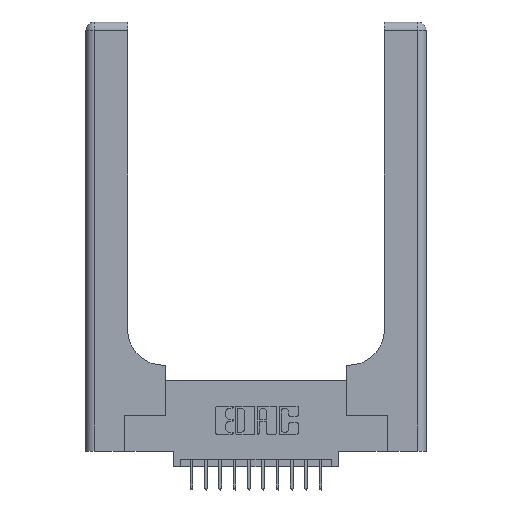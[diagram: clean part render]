
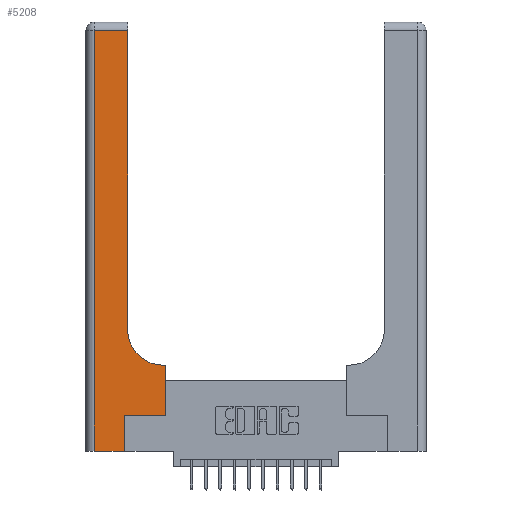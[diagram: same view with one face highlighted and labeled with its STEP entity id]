
A CAD part, top view. The second image highlights one B-rep face of the part: STEP entity #5208.
In plain terms, the highlighted planar face has unit normal (0, 0, 1).
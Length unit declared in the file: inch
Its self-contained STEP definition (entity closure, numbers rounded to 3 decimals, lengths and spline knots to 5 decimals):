
#75 = VERTEX_POINT ( 'NONE', #4749 ) ;
#174 = CARTESIAN_POINT ( 'NONE',  ( 0.5415, 0.6, 0.37 ) ) ;
#355 = PLANE ( 'NONE',  #7855 ) ;
#551 = CARTESIAN_POINT ( 'NONE',  ( 0.269, 0.25, 0.37 ) ) ;
#802 = EDGE_LOOP ( 'NONE', ( #6903, #7580, #8906, #9779, #12419, #13769, #14376, #15726, #12023 ) ) ;
#1086 = VERTEX_POINT ( 'NONE', #11250 ) ;
#1404 = EDGE_CURVE ( 'NONE', #2986, #9551, #2922, .T. ) ;
#1509 = CARTESIAN_POINT ( 'NONE',  ( 0.06, 2.94, 0.37 ) ) ;
#1578 = DIRECTION ( 'NONE',  ( -1., 0., 0. ) ) ;
#1774 = DIRECTION ( 'NONE',  ( 0., 0., -1. ) ) ;
#1851 = DIRECTION ( 'NONE',  ( 0., -1., 0. ) ) ;
#2357 = CARTESIAN_POINT ( 'NONE',  ( 0.2915, 2.94, 0.37 ) ) ;
#2883 = CARTESIAN_POINT ( 'NONE',  ( 0.269, 0.25, 0.37 ) ) ;
#2922 = LINE ( 'NONE', #15403, #3370 ) ;
#2986 = VERTEX_POINT ( 'NONE', #9006 ) ;
#3007 = LINE ( 'NONE', #17312, #10222 ) ;
#3303 = CARTESIAN_POINT ( 'NONE',  ( 0., 2.94, 0.37 ) ) ;
#3370 = VECTOR ( 'NONE', #14611, 39.37008 ) ;
#3864 = LINE ( 'NONE', #2883, #14214 ) ;
#3931 = EDGE_CURVE ( 'NONE', #75, #1086, #3007, .T. ) ;
#3934 = LINE ( 'NONE', #11621, #7104 ) ;
#4386 = EDGE_CURVE ( 'NONE', #4642, #75, #3864, .T. ) ;
#4631 = VECTOR ( 'NONE', #11720, 39.37008 ) ;
#4642 = VERTEX_POINT ( 'NONE', #551 ) ;
#4749 = CARTESIAN_POINT ( 'NONE',  ( 0.5585, 0.25, 0.37 ) ) ;
#4827 = VECTOR ( 'NONE', #1851, 39.37008 ) ;
#5066 = LINE ( 'NONE', #10363, #4631 ) ;
#5208 = ADVANCED_FACE ( 'NONE', ( #13985 ), #355, .F. ) ;
#6571 = VECTOR ( 'NONE', #1578, 39.37008 ) ;
#6903 = ORIENTED_EDGE ( 'NONE', *, *, #11192, .T. ) ;
#7104 = VECTOR ( 'NONE', #14263, 39.37008 ) ;
#7114 = CARTESIAN_POINT ( 'NONE',  ( 0.5415, 0.85, 0.37 ) ) ;
#7189 = VERTEX_POINT ( 'NONE', #1509 ) ;
#7580 = ORIENTED_EDGE ( 'NONE', *, *, #11740, .T. ) ;
#7855 = AXIS2_PLACEMENT_3D ( 'NONE', #9987, #1774, #11363 ) ;
#8466 = DIRECTION ( 'NONE',  ( 1., 0., 0. ) ) ;
#8906 = ORIENTED_EDGE ( 'NONE', *, *, #12664, .T. ) ;
#8996 = CARTESIAN_POINT ( 'NONE',  ( 0.2915, 0.85, 0.37 ) ) ;
#9006 = CARTESIAN_POINT ( 'NONE',  ( 0.06, 0., 0.37 ) ) ;
#9551 = VERTEX_POINT ( 'NONE', #16705 ) ;
#9715 = DIRECTION ( 'NONE',  ( 1., 0., 0. ) ) ;
#9779 = ORIENTED_EDGE ( 'NONE', *, *, #1404, .T. ) ;
#9987 = CARTESIAN_POINT ( 'NONE',  ( 0., 3., 0.37 ) ) ;
#10138 = LINE ( 'NONE', #15151, #6571 ) ;
#10222 = VECTOR ( 'NONE', #17173, 39.37008 ) ;
#10363 = CARTESIAN_POINT ( 'NONE',  ( 0.2915, 3., 0.37 ) ) ;
#10376 = EDGE_CURVE ( 'NONE', #1086, #10419, #10138, .T. ) ;
#10419 = VERTEX_POINT ( 'NONE', #174 ) ;
#11001 = AXIS2_PLACEMENT_3D ( 'NONE', #7114, #16471, #8466 ) ;
#11192 = EDGE_CURVE ( 'NONE', #11193, #14089, #5066, .T. ) ;
#11193 = VERTEX_POINT ( 'NONE', #8996 ) ;
#11250 = CARTESIAN_POINT ( 'NONE',  ( 0.5585, 0.6, 0.37 ) ) ;
#11363 = DIRECTION ( 'NONE',  ( -1., 0., 0. ) ) ;
#11378 = VECTOR ( 'NONE', #12788, 39.37008 ) ;
#11431 = CARTESIAN_POINT ( 'NONE',  ( 0.06, 3., 0.37 ) ) ;
#11621 = CARTESIAN_POINT ( 'NONE',  ( 0.269, 0., 0.37 ) ) ;
#11720 = DIRECTION ( 'NONE',  ( 0., 1., 0. ) ) ;
#11740 = EDGE_CURVE ( 'NONE', #14089, #7189, #11772, .T. ) ;
#11772 = LINE ( 'NONE', #3303, #11378 ) ;
#11976 = LINE ( 'NONE', #11431, #4827 ) ;
#12023 = ORIENTED_EDGE ( 'NONE', *, *, #14438, .T. ) ;
#12419 = ORIENTED_EDGE ( 'NONE', *, *, #12430, .T. ) ;
#12430 = EDGE_CURVE ( 'NONE', #9551, #4642, #3934, .T. ) ;
#12664 = EDGE_CURVE ( 'NONE', #7189, #2986, #11976, .T. ) ;
#12788 = DIRECTION ( 'NONE',  ( -1., 0., 0. ) ) ;
#13769 = ORIENTED_EDGE ( 'NONE', *, *, #4386, .T. ) ;
#13985 = FACE_OUTER_BOUND ( 'NONE', #802, .T. ) ;
#14089 = VERTEX_POINT ( 'NONE', #2357 ) ;
#14214 = VECTOR ( 'NONE', #9715, 39.37008 ) ;
#14263 = DIRECTION ( 'NONE',  ( 0., 1., 0. ) ) ;
#14376 = ORIENTED_EDGE ( 'NONE', *, *, #3931, .T. ) ;
#14438 = EDGE_CURVE ( 'NONE', #10419, #11193, #14446, .T. ) ;
#14446 = CIRCLE ( 'NONE', #11001, 0.25 ) ;
#14611 = DIRECTION ( 'NONE',  ( 1., 0., 0. ) ) ;
#15151 = CARTESIAN_POINT ( 'NONE',  ( 0.2915, 0.6, 0.37 ) ) ;
#15403 = CARTESIAN_POINT ( 'NONE',  ( 0., 0., 0.37 ) ) ;
#15726 = ORIENTED_EDGE ( 'NONE', *, *, #10376, .T. ) ;
#16471 = DIRECTION ( 'NONE',  ( 0., 0., -1. ) ) ;
#16705 = CARTESIAN_POINT ( 'NONE',  ( 0.269, 0., 0.37 ) ) ;
#17173 = DIRECTION ( 'NONE',  ( 0., 1., 0. ) ) ;
#17312 = CARTESIAN_POINT ( 'NONE',  ( 0.5585, 0.25, 0.37 ) ) ;
